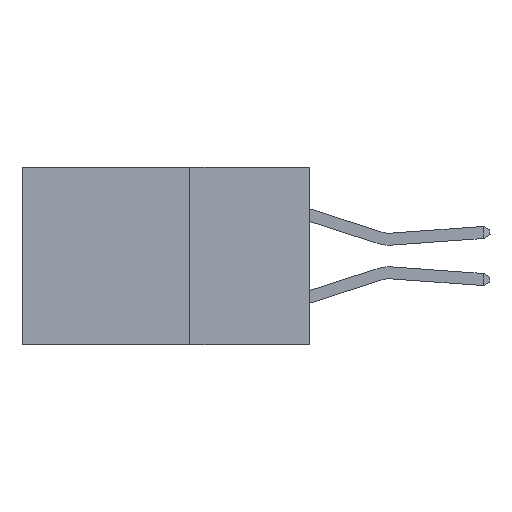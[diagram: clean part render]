
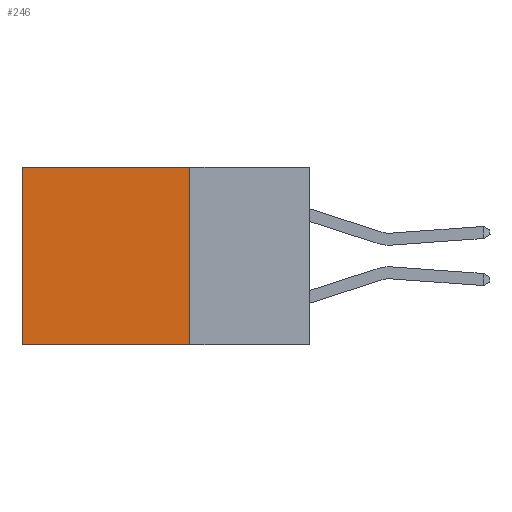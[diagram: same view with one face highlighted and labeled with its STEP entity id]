
A CAD part, left-side view. The second image highlights one B-rep face of the part: STEP entity #246.
In plain terms, the highlighted planar face has unit normal (-1, 0, 0).
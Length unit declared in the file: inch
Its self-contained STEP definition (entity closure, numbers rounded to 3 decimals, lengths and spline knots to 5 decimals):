
#44 = ORIENTED_EDGE ( 'NONE', *, *, #2054, .T. ) ;
#215 = VECTOR ( 'NONE', #1559, 39.37008 ) ;
#246 = ADVANCED_FACE ( 'NONE', ( #11978 ), #4041, .F. ) ;
#286 = DIRECTION ( 'NONE',  ( 0., 0., -1. ) ) ;
#339 = AXIS2_PLACEMENT_3D ( 'NONE', #3087, #6913, #10700 ) ;
#600 = VECTOR ( 'NONE', #4512, 39.37008 ) ;
#653 = ORIENTED_EDGE ( 'NONE', *, *, #8519, .T. ) ;
#701 = CARTESIAN_POINT ( 'NONE',  ( 0.2615, 0.6, -0.37 ) ) ;
#739 = CARTESIAN_POINT ( 'NONE',  ( 0.2615, 0.25, -0.37 ) ) ;
#1230 = LINE ( 'NONE', #1610, #600 ) ;
#1297 = CARTESIAN_POINT ( 'NONE',  ( 0.2615, 0.6, 0. ) ) ;
#1559 = DIRECTION ( 'NONE',  ( 0., 1., 0. ) ) ;
#1610 = CARTESIAN_POINT ( 'NONE',  ( 0.2615, 0.25, 0. ) ) ;
#1632 = EDGE_CURVE ( 'NONE', #2721, #10112, #2107, .T. ) ;
#1982 = ORIENTED_EDGE ( 'NONE', *, *, #1632, .F. ) ;
#2054 = EDGE_CURVE ( 'NONE', #3377, #9584, #10018, .T. ) ;
#2107 = LINE ( 'NONE', #7047, #9462 ) ;
#2721 = VERTEX_POINT ( 'NONE', #10715 ) ;
#2802 = CARTESIAN_POINT ( 'NONE',  ( 0.2615, 0.6, -0.37 ) ) ;
#3087 = CARTESIAN_POINT ( 'NONE',  ( 0.2615, 0.25, -0.37 ) ) ;
#3377 = VERTEX_POINT ( 'NONE', #1297 ) ;
#4041 = PLANE ( 'NONE',  #339 ) ;
#4512 = DIRECTION ( 'NONE',  ( 0., 1., 0. ) ) ;
#4938 = VECTOR ( 'NONE', #8541, 39.37008 ) ;
#5356 = LINE ( 'NONE', #12025, #215 ) ;
#6124 = ORIENTED_EDGE ( 'NONE', *, *, #6544, .F. ) ;
#6355 = EDGE_LOOP ( 'NONE', ( #44, #6124, #1982, #653 ) ) ;
#6544 = EDGE_CURVE ( 'NONE', #10112, #9584, #5356, .T. ) ;
#6913 = DIRECTION ( 'NONE',  ( 1., 0., 0. ) ) ;
#7047 = CARTESIAN_POINT ( 'NONE',  ( 0.2615, 0.25, -0.37 ) ) ;
#8519 = EDGE_CURVE ( 'NONE', #2721, #3377, #1230, .T. ) ;
#8541 = DIRECTION ( 'NONE',  ( 0., 0., -1. ) ) ;
#9462 = VECTOR ( 'NONE', #286, 39.37008 ) ;
#9584 = VERTEX_POINT ( 'NONE', #701 ) ;
#10018 = LINE ( 'NONE', #2802, #4938 ) ;
#10112 = VERTEX_POINT ( 'NONE', #739 ) ;
#10700 = DIRECTION ( 'NONE',  ( 0., 0., -1. ) ) ;
#10715 = CARTESIAN_POINT ( 'NONE',  ( 0.2615, 0.25, 0. ) ) ;
#11978 = FACE_OUTER_BOUND ( 'NONE', #6355, .T. ) ;
#12025 = CARTESIAN_POINT ( 'NONE',  ( 0.2615, 0.25, -0.37 ) ) ;
